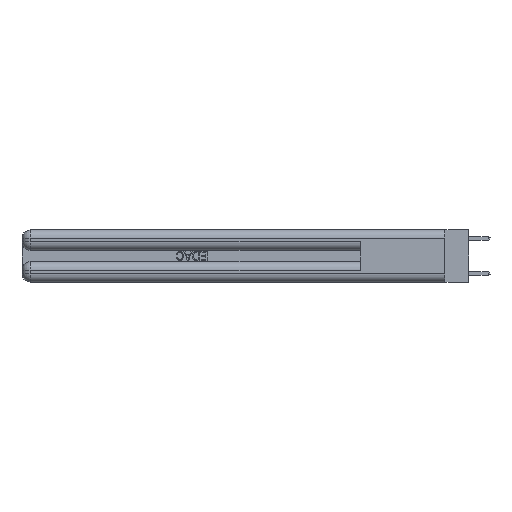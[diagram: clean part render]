
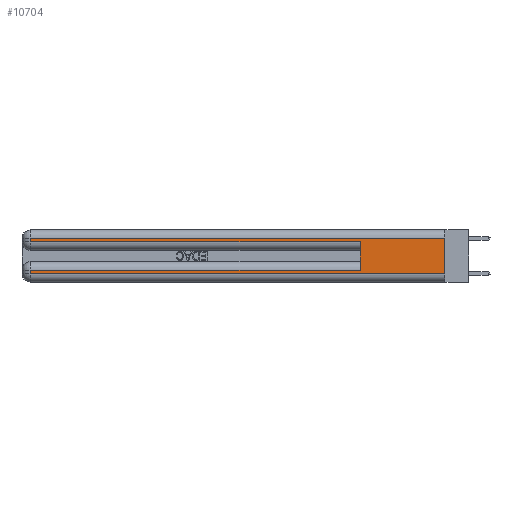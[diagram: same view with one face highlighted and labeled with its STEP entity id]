
A CAD part, left-side view. The second image highlights one B-rep face of the part: STEP entity #10704.
In plain terms, the highlighted planar face has unit normal (-1, 0, 0).
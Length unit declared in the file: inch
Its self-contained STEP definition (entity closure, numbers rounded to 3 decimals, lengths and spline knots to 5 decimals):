
#129 = EDGE_LOOP ( 'NONE', ( #24951, #26504, #25870, #6838, #25319, #7298, #18476, #1104 ) ) ;
#349 = CARTESIAN_POINT ( 'NONE',  ( 0., 2.94, 0.31 ) ) ;
#640 = LINE ( 'NONE', #16508, #20071 ) ;
#868 = CARTESIAN_POINT ( 'NONE',  ( 0., 2.94, 0.06 ) ) ;
#916 = CARTESIAN_POINT ( 'NONE',  ( 0., 0.6, 0.285 ) ) ;
#1104 = ORIENTED_EDGE ( 'NONE', *, *, #7279, .T. ) ;
#2075 = LINE ( 'NONE', #28981, #25882 ) ;
#2841 = VECTOR ( 'NONE', #17456, 39.37008 ) ;
#2916 = VERTEX_POINT ( 'NONE', #17585 ) ;
#3478 = EDGE_CURVE ( 'NONE', #28325, #21668, #640, .T. ) ;
#3949 = CARTESIAN_POINT ( 'NONE',  ( 0., 0., 0.37 ) ) ;
#4208 = DIRECTION ( 'NONE',  ( 0., 0., -1. ) ) ;
#4672 = LINE ( 'NONE', #13610, #5753 ) ;
#5753 = VECTOR ( 'NONE', #7437, 39.37008 ) ;
#5838 = DIRECTION ( 'NONE',  ( 0., 0., 1. ) ) ;
#6158 = EDGE_CURVE ( 'NONE', #2916, #8133, #26424, .T. ) ;
#6838 = ORIENTED_EDGE ( 'NONE', *, *, #10835, .T. ) ;
#6931 = VECTOR ( 'NONE', #4208, 39.37008 ) ;
#7091 = CARTESIAN_POINT ( 'NONE',  ( 0., 0., 0.06 ) ) ;
#7241 = VERTEX_POINT ( 'NONE', #7091 ) ;
#7279 = EDGE_CURVE ( 'NONE', #19098, #7241, #25453, .T. ) ;
#7298 = ORIENTED_EDGE ( 'NONE', *, *, #3478, .T. ) ;
#7437 = DIRECTION ( 'NONE',  ( 0., -1., 0. ) ) ;
#7598 = EDGE_CURVE ( 'NONE', #21668, #19098, #2075, .T. ) ;
#8133 = VERTEX_POINT ( 'NONE', #349 ) ;
#8145 = CARTESIAN_POINT ( 'NONE',  ( 0., 0.6, 0.085 ) ) ;
#8593 = DIRECTION ( 'NONE',  ( 0., 0., -1. ) ) ;
#8771 = FACE_OUTER_BOUND ( 'NONE', #129, .T. ) ;
#10000 = VECTOR ( 'NONE', #8593, 39.37008 ) ;
#10445 = AXIS2_PLACEMENT_3D ( 'NONE', #3949, #15105, #18030 ) ;
#10704 = ADVANCED_FACE ( 'NONE', ( #8771 ), #17590, .F. ) ;
#10835 = EDGE_CURVE ( 'NONE', #12917, #28653, #4672, .T. ) ;
#11212 = EDGE_CURVE ( 'NONE', #2916, #7241, #19489, .T. ) ;
#12258 = CARTESIAN_POINT ( 'NONE',  ( 0., 2.94, 0.085 ) ) ;
#12917 = VERTEX_POINT ( 'NONE', #22894 ) ;
#13151 = CARTESIAN_POINT ( 'NONE',  ( 0., 2.94, 0.37 ) ) ;
#13610 = CARTESIAN_POINT ( 'NONE',  ( 0., 0., 0.285 ) ) ;
#15105 = DIRECTION ( 'NONE',  ( 1., 0., 0. ) ) ;
#15110 = CARTESIAN_POINT ( 'NONE',  ( 0., 0., 0.31 ) ) ;
#16482 = CARTESIAN_POINT ( 'NONE',  ( 0., 0., 0.06 ) ) ;
#16508 = CARTESIAN_POINT ( 'NONE',  ( 0., 0., 0.085 ) ) ;
#16998 = LINE ( 'NONE', #28321, #25104 ) ;
#17456 = DIRECTION ( 'NONE',  ( 0., 1., 0. ) ) ;
#17585 = CARTESIAN_POINT ( 'NONE',  ( 0., 0., 0.31 ) ) ;
#17590 = PLANE ( 'NONE',  #10445 ) ;
#18030 = DIRECTION ( 'NONE',  ( 0., 0., -1. ) ) ;
#18198 = DIRECTION ( 'NONE',  ( 0., 0., -1. ) ) ;
#18476 = ORIENTED_EDGE ( 'NONE', *, *, #7598, .T. ) ;
#19098 = VERTEX_POINT ( 'NONE', #868 ) ;
#19489 = LINE ( 'NONE', #24316, #10000 ) ;
#20071 = VECTOR ( 'NONE', #27688, 39.37008 ) ;
#21267 = EDGE_CURVE ( 'NONE', #8133, #12917, #23632, .T. ) ;
#21668 = VERTEX_POINT ( 'NONE', #12258 ) ;
#22894 = CARTESIAN_POINT ( 'NONE',  ( 0., 2.94, 0.285 ) ) ;
#22944 = DIRECTION ( 'NONE',  ( 0., -1., 0. ) ) ;
#23042 = VECTOR ( 'NONE', #22944, 39.37008 ) ;
#23632 = LINE ( 'NONE', #13151, #6931 ) ;
#24316 = CARTESIAN_POINT ( 'NONE',  ( 0., 0., 0.37 ) ) ;
#24868 = EDGE_CURVE ( 'NONE', #28325, #28653, #16998, .T. ) ;
#24951 = ORIENTED_EDGE ( 'NONE', *, *, #11212, .F. ) ;
#25104 = VECTOR ( 'NONE', #5838, 39.37008 ) ;
#25319 = ORIENTED_EDGE ( 'NONE', *, *, #24868, .F. ) ;
#25453 = LINE ( 'NONE', #16482, #23042 ) ;
#25870 = ORIENTED_EDGE ( 'NONE', *, *, #21267, .T. ) ;
#25882 = VECTOR ( 'NONE', #18198, 39.37008 ) ;
#26424 = LINE ( 'NONE', #15110, #2841 ) ;
#26504 = ORIENTED_EDGE ( 'NONE', *, *, #6158, .T. ) ;
#27688 = DIRECTION ( 'NONE',  ( 0., 1., 0. ) ) ;
#28321 = CARTESIAN_POINT ( 'NONE',  ( 0., 0.6, 0.145 ) ) ;
#28325 = VERTEX_POINT ( 'NONE', #8145 ) ;
#28653 = VERTEX_POINT ( 'NONE', #916 ) ;
#28981 = CARTESIAN_POINT ( 'NONE',  ( 0., 2.94, 0.37 ) ) ;
